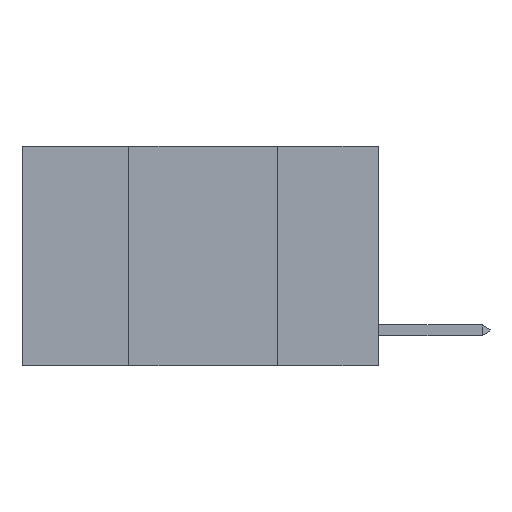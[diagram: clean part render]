
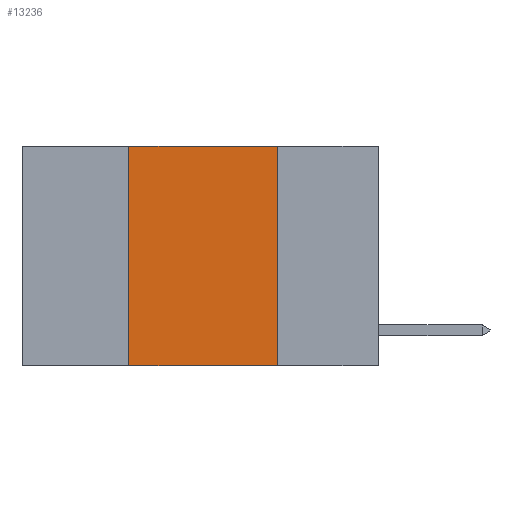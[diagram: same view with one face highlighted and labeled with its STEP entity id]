
A CAD part, left-side view. The second image highlights one B-rep face of the part: STEP entity #13236.
In plain terms, the highlighted planar face has unit normal (-1, 0, 0).
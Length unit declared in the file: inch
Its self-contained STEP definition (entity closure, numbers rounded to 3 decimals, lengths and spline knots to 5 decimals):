
#543 = CARTESIAN_POINT ( 'NONE',  ( 0., 0.17, 0. ) ) ;
#2393 = EDGE_CURVE ( 'NONE', #15976, #13516, #17065, .T. ) ;
#3895 = AXIS2_PLACEMENT_3D ( 'NONE', #16435, #8916, #16260 ) ;
#3986 = CARTESIAN_POINT ( 'NONE',  ( 0., 0.42, -0.37 ) ) ;
#4359 = DIRECTION ( 'NONE',  ( 0., 0., 1. ) ) ;
#4930 = FACE_OUTER_BOUND ( 'NONE', #18336, .T. ) ;
#5418 = VERTEX_POINT ( 'NONE', #3986 ) ;
#5812 = VECTOR ( 'NONE', #9215, 39.37008 ) ;
#6329 = VECTOR ( 'NONE', #4359, 39.37008 ) ;
#7040 = DIRECTION ( 'NONE',  ( 0., -1., 0. ) ) ;
#7304 = PLANE ( 'NONE',  #3895 ) ;
#8121 = ORIENTED_EDGE ( 'NONE', *, *, #9531, .F. ) ;
#8286 = ORIENTED_EDGE ( 'NONE', *, *, #13204, .T. ) ;
#8916 = DIRECTION ( 'NONE',  ( 1., 0., 0. ) ) ;
#9215 = DIRECTION ( 'NONE',  ( 0., -1., 0. ) ) ;
#9498 = CARTESIAN_POINT ( 'NONE',  ( 0., 0.17, -0.37 ) ) ;
#9531 = EDGE_CURVE ( 'NONE', #5418, #15976, #10260, .T. ) ;
#10260 = LINE ( 'NONE', #14918, #6329 ) ;
#12753 = LINE ( 'NONE', #14396, #14831 ) ;
#12816 = CARTESIAN_POINT ( 'NONE',  ( 0., 0.42, 0. ) ) ;
#13204 = EDGE_CURVE ( 'NONE', #5418, #14793, #12753, .T. ) ;
#13236 = ADVANCED_FACE ( 'NONE', ( #4930 ), #7304, .F. ) ;
#13303 = ORIENTED_EDGE ( 'NONE', *, *, #2393, .F. ) ;
#13516 = VERTEX_POINT ( 'NONE', #543 ) ;
#13721 = CARTESIAN_POINT ( 'NONE',  ( 0., 0.6, 0. ) ) ;
#14396 = CARTESIAN_POINT ( 'NONE',  ( 0., 0.6, -0.37 ) ) ;
#14793 = VERTEX_POINT ( 'NONE', #9498 ) ;
#14831 = VECTOR ( 'NONE', #7040, 39.37008 ) ;
#14892 = EDGE_CURVE ( 'NONE', #13516, #14793, #15001, .T. ) ;
#14918 = CARTESIAN_POINT ( 'NONE',  ( 0., 0.42, 0. ) ) ;
#15001 = LINE ( 'NONE', #16168, #16814 ) ;
#15976 = VERTEX_POINT ( 'NONE', #12816 ) ;
#16039 = DIRECTION ( 'NONE',  ( 0., 0., -1. ) ) ;
#16168 = CARTESIAN_POINT ( 'NONE',  ( 0., 0.17, 0. ) ) ;
#16260 = DIRECTION ( 'NONE',  ( 0., 0., -1. ) ) ;
#16435 = CARTESIAN_POINT ( 'NONE',  ( 0., 0.6, 0. ) ) ;
#16814 = VECTOR ( 'NONE', #16039, 39.37008 ) ;
#17065 = LINE ( 'NONE', #13721, #5812 ) ;
#18336 = EDGE_LOOP ( 'NONE', ( #18539, #13303, #8121, #8286 ) ) ;
#18539 = ORIENTED_EDGE ( 'NONE', *, *, #14892, .F. ) ;
